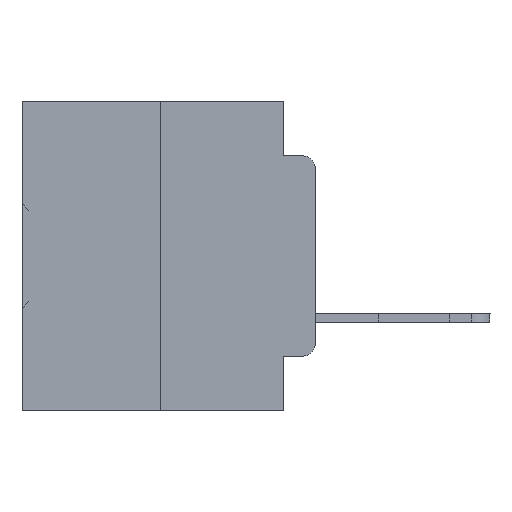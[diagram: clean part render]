
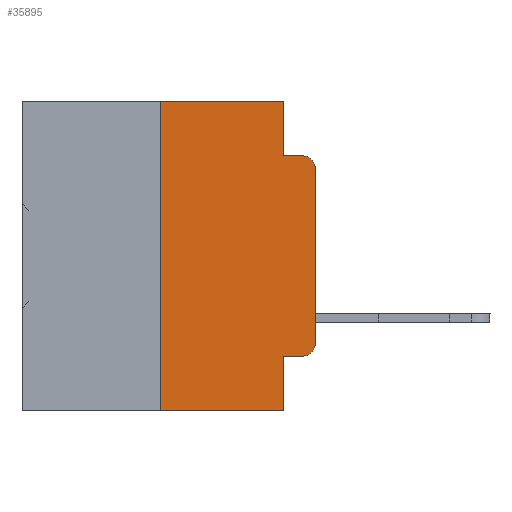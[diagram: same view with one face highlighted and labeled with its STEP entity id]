
A CAD part, left-side view. The second image highlights one B-rep face of the part: STEP entity #35895.
In plain terms, the highlighted planar face has unit normal (-1, 0, 0).
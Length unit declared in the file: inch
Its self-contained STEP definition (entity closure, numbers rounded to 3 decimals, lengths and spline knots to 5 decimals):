
#1590 = DIRECTION ( 'NONE',  ( 0., 0., -1. ) ) ;
#2248 = DIRECTION ( 'NONE',  ( 0., 0., -1. ) ) ;
#3443 = CARTESIAN_POINT ( 'NONE',  ( 0., 0., -0.1085 ) ) ;
#3507 = AXIS2_PLACEMENT_3D ( 'NONE', #31384, #28500, #2248 ) ;
#3672 = EDGE_CURVE ( 'NONE', #32894, #20793, #24983, .T. ) ;
#3736 = EDGE_CURVE ( 'NONE', #9648, #7913, #4466, .T. ) ;
#4357 = VECTOR ( 'NONE', #15292, 39.37008 ) ;
#4466 = LINE ( 'NONE', #16156, #7703 ) ;
#4799 = CARTESIAN_POINT ( 'NONE',  ( 0., 0.051, 0. ) ) ;
#5374 = EDGE_CURVE ( 'NONE', #32894, #31978, #27729, .T. ) ;
#5407 = ORIENTED_EDGE ( 'NONE', *, *, #3736, .T. ) ;
#5615 = ORIENTED_EDGE ( 'NONE', *, *, #10269, .T. ) ;
#5670 = CARTESIAN_POINT ( 'NONE',  ( 0., 0.051, -0.0885 ) ) ;
#6326 = LINE ( 'NONE', #12078, #20445 ) ;
#6426 = VERTEX_POINT ( 'NONE', #25643 ) ;
#7038 = CARTESIAN_POINT ( 'NONE',  ( 0., 0.051, 0. ) ) ;
#7201 = CIRCLE ( 'NONE', #3507, 0.02 ) ;
#7457 = CARTESIAN_POINT ( 'NONE',  ( 0., 0.051, -0.0885 ) ) ;
#7703 = VECTOR ( 'NONE', #30910, 39.37008 ) ;
#7913 = VERTEX_POINT ( 'NONE', #3443 ) ;
#8364 = DIRECTION ( 'NONE',  ( 0., -1., 0. ) ) ;
#9648 = VERTEX_POINT ( 'NONE', #18164 ) ;
#10235 = CARTESIAN_POINT ( 'NONE',  ( 0., 0.02, -0.1085 ) ) ;
#10269 = EDGE_CURVE ( 'NONE', #7913, #29683, #28460, .T. ) ;
#10756 = VERTEX_POINT ( 'NONE', #14739 ) ;
#11039 = CARTESIAN_POINT ( 'NONE',  ( 0., 0.473, 0. ) ) ;
#11720 = VERTEX_POINT ( 'NONE', #4799 ) ;
#11954 = AXIS2_PLACEMENT_3D ( 'NONE', #10235, #27852, #1590 ) ;
#12078 = CARTESIAN_POINT ( 'NONE',  ( 0., 0.25, 0. ) ) ;
#12402 = DIRECTION ( 'NONE',  ( 0., 0., -1. ) ) ;
#12678 = VERTEX_POINT ( 'NONE', #7457 ) ;
#12873 = EDGE_LOOP ( 'NONE', ( #5407, #5615, #24516, #23745, #35791, #34489, #37019, #17421, #23223, #13796 ) ) ;
#13234 = VECTOR ( 'NONE', #24800, 39.37008 ) ;
#13796 = ORIENTED_EDGE ( 'NONE', *, *, #21958, .T. ) ;
#14126 = EDGE_CURVE ( 'NONE', #10756, #11720, #19718, .T. ) ;
#14739 = CARTESIAN_POINT ( 'NONE',  ( 0., 0.25, 0. ) ) ;
#15292 = DIRECTION ( 'NONE',  ( 0., -1., 0. ) ) ;
#16156 = CARTESIAN_POINT ( 'NONE',  ( 0., 0., 0. ) ) ;
#17421 = ORIENTED_EDGE ( 'NONE', *, *, #5374, .F. ) ;
#17636 = DIRECTION ( 'NONE',  ( 0., 0., 1. ) ) ;
#18164 = CARTESIAN_POINT ( 'NONE',  ( 0., 0., -0.3915 ) ) ;
#19194 = CARTESIAN_POINT ( 'NONE',  ( 0., 0.02, -0.0885 ) ) ;
#19718 = LINE ( 'NONE', #28134, #20336 ) ;
#20056 = DIRECTION ( 'NONE',  ( 1., 0., 0. ) ) ;
#20336 = VECTOR ( 'NONE', #27593, 39.37008 ) ;
#20445 = VECTOR ( 'NONE', #17636, 39.37008 ) ;
#20793 = VERTEX_POINT ( 'NONE', #34816 ) ;
#21958 = EDGE_CURVE ( 'NONE', #20793, #9648, #7201, .T. ) ;
#22558 = FACE_OUTER_BOUND ( 'NONE', #12873, .T. ) ;
#23138 = CARTESIAN_POINT ( 'NONE',  ( 0., 0.051, -0.4115 ) ) ;
#23223 = ORIENTED_EDGE ( 'NONE', *, *, #3672, .T. ) ;
#23406 = EDGE_CURVE ( 'NONE', #11720, #12678, #24013, .T. ) ;
#23503 = LINE ( 'NONE', #5670, #30712 ) ;
#23535 = AXIS2_PLACEMENT_3D ( 'NONE', #11039, #20056, #34239 ) ;
#23745 = ORIENTED_EDGE ( 'NONE', *, *, #23406, .F. ) ;
#24013 = LINE ( 'NONE', #30136, #26776 ) ;
#24516 = ORIENTED_EDGE ( 'NONE', *, *, #27197, .F. ) ;
#24800 = DIRECTION ( 'NONE',  ( 0., -1., 0. ) ) ;
#24983 = LINE ( 'NONE', #30532, #13234 ) ;
#25643 = CARTESIAN_POINT ( 'NONE',  ( 0., 0.25, -0.5 ) ) ;
#26776 = VECTOR ( 'NONE', #29748, 39.37008 ) ;
#27197 = EDGE_CURVE ( 'NONE', #12678, #29683, #23503, .T. ) ;
#27593 = DIRECTION ( 'NONE',  ( 0., -1., 0. ) ) ;
#27729 = LINE ( 'NONE', #7038, #28269 ) ;
#27852 = DIRECTION ( 'NONE',  ( -1., 0., 0. ) ) ;
#28102 = PLANE ( 'NONE',  #23535 ) ;
#28134 = CARTESIAN_POINT ( 'NONE',  ( 0., 0.473, 0. ) ) ;
#28269 = VECTOR ( 'NONE', #12402, 39.37008 ) ;
#28460 = CIRCLE ( 'NONE', #11954, 0.02 ) ;
#28500 = DIRECTION ( 'NONE',  ( -1., 0., 0. ) ) ;
#29683 = VERTEX_POINT ( 'NONE', #19194 ) ;
#29748 = DIRECTION ( 'NONE',  ( 0., 0., -1. ) ) ;
#30136 = CARTESIAN_POINT ( 'NONE',  ( 0., 0.051, 0. ) ) ;
#30532 = CARTESIAN_POINT ( 'NONE',  ( 0., 0.051, -0.4115 ) ) ;
#30712 = VECTOR ( 'NONE', #8364, 39.37008 ) ;
#30910 = DIRECTION ( 'NONE',  ( 0., 0., 1. ) ) ;
#31293 = EDGE_CURVE ( 'NONE', #6426, #31978, #32735, .T. ) ;
#31384 = CARTESIAN_POINT ( 'NONE',  ( 0., 0.02, -0.3915 ) ) ;
#31978 = VERTEX_POINT ( 'NONE', #34575 ) ;
#32735 = LINE ( 'NONE', #32923, #4357 ) ;
#32894 = VERTEX_POINT ( 'NONE', #23138 ) ;
#32923 = CARTESIAN_POINT ( 'NONE',  ( 0., 0.473, -0.5 ) ) ;
#34239 = DIRECTION ( 'NONE',  ( 0., 0., -1. ) ) ;
#34489 = ORIENTED_EDGE ( 'NONE', *, *, #35115, .F. ) ;
#34575 = CARTESIAN_POINT ( 'NONE',  ( 0., 0.051, -0.5 ) ) ;
#34816 = CARTESIAN_POINT ( 'NONE',  ( 0., 0.02, -0.4115 ) ) ;
#35115 = EDGE_CURVE ( 'NONE', #6426, #10756, #6326, .T. ) ;
#35791 = ORIENTED_EDGE ( 'NONE', *, *, #14126, .F. ) ;
#35895 = ADVANCED_FACE ( 'NONE', ( #22558 ), #28102, .F. ) ;
#37019 = ORIENTED_EDGE ( 'NONE', *, *, #31293, .T. ) ;
